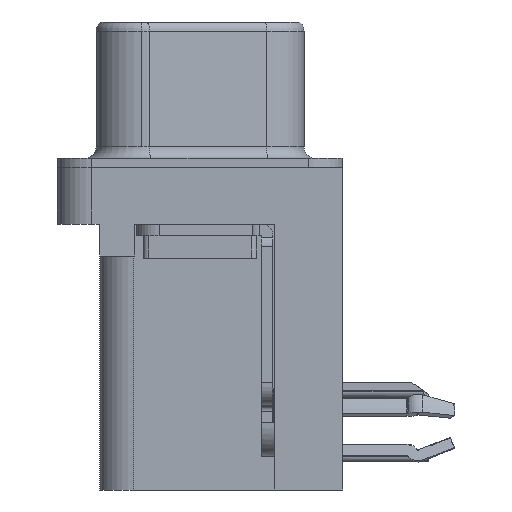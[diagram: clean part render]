
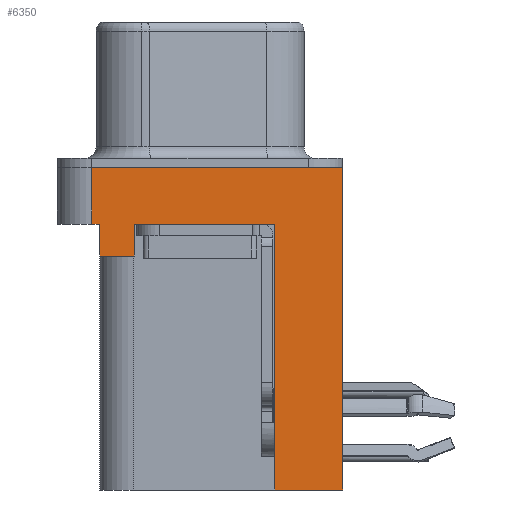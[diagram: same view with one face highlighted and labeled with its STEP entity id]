
A CAD part, left-side view. The second image highlights one B-rep face of the part: STEP entity #6350.
In plain terms, the highlighted planar face has unit normal (-1, 0, 0).
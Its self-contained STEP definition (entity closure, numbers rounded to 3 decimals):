
#9 = VECTOR ( 'NONE', #6792, 1000. ) ;
#83 = VECTOR ( 'NONE', #28165, 1000. ) ;
#802 = ORIENTED_EDGE ( 'NONE', *, *, #1730, .F. ) ;
#912 = DIRECTION ( 'NONE',  ( 0., 0., 1. ) ) ;
#996 = VECTOR ( 'NONE', #2205, 1000. ) ;
#1730 = EDGE_CURVE ( 'NONE', #5535, #6519, #18132, .T. ) ;
#1905 = VERTEX_POINT ( 'NONE', #10035 ) ;
#2050 = VECTOR ( 'NONE', #21379, 1000. ) ;
#2205 = DIRECTION ( 'NONE',  ( 0., 0., 1. ) ) ;
#2220 = ORIENTED_EDGE ( 'NONE', *, *, #10463, .F. ) ;
#2523 = CARTESIAN_POINT ( 'NONE',  ( -2.91, -6.275, -2.5 ) ) ;
#2589 = VECTOR ( 'NONE', #27114, 1000. ) ;
#3514 = EDGE_CURVE ( 'NONE', #9556, #25542, #28544, .T. ) ;
#4251 = CARTESIAN_POINT ( 'NONE',  ( -2.91, 2.895, -3.9 ) ) ;
#4475 = EDGE_CURVE ( 'NONE', #10401, #25542, #5679, .T. ) ;
#4551 = DIRECTION ( 'NONE',  ( -1., 0., 0. ) ) ;
#4852 = VECTOR ( 'NONE', #25044, 1000. ) ;
#5535 = VERTEX_POINT ( 'NONE', #4251 ) ;
#5679 = LINE ( 'NONE', #17106, #11137 ) ;
#5737 = VECTOR ( 'NONE', #26136, 1000. ) ;
#5828 = EDGE_CURVE ( 'NONE', #21570, #10401, #19045, .T. ) ;
#6350 = ADVANCED_FACE ( 'NONE', ( #22339 ), #6562, .T. ) ;
#6415 = DIRECTION ( 'NONE',  ( 0., 0., 1. ) ) ;
#6519 = VERTEX_POINT ( 'NONE', #11495 ) ;
#6562 = PLANE ( 'NONE',  #12569 ) ;
#6792 = DIRECTION ( 'NONE',  ( 0., 1., 0. ) ) ;
#6856 = CARTESIAN_POINT ( 'NONE',  ( -2.91, -6.275, -2.5 ) ) ;
#8208 = LINE ( 'NONE', #27894, #2050 ) ;
#9449 = ORIENTED_EDGE ( 'NONE', *, *, #3514, .T. ) ;
#9556 = VERTEX_POINT ( 'NONE', #10599 ) ;
#9736 = CARTESIAN_POINT ( 'NONE',  ( -2.91, 2.895, -3.9 ) ) ;
#10035 = CARTESIAN_POINT ( 'NONE',  ( -2.91, -3.295, -14.2 ) ) ;
#10401 = VERTEX_POINT ( 'NONE', #12692 ) ;
#10463 = EDGE_CURVE ( 'NONE', #1905, #11185, #8208, .T. ) ;
#10571 = EDGE_CURVE ( 'NONE', #6519, #11316, #28325, .T. ) ;
#10599 = CARTESIAN_POINT ( 'NONE',  ( -2.91, -6.275, -14.2 ) ) ;
#11058 = LINE ( 'NONE', #6856, #21261 ) ;
#11137 = VECTOR ( 'NONE', #14369, 1000. ) ;
#11185 = VERTEX_POINT ( 'NONE', #17406 ) ;
#11316 = VERTEX_POINT ( 'NONE', #15526 ) ;
#11495 = CARTESIAN_POINT ( 'NONE',  ( -2.91, 4.425, -3.9 ) ) ;
#11785 = ORIENTED_EDGE ( 'NONE', *, *, #21209, .F. ) ;
#12230 = ORIENTED_EDGE ( 'NONE', *, *, #15459, .T. ) ;
#12569 = AXIS2_PLACEMENT_3D ( 'NONE', #2523, #4551, #6415 ) ;
#12682 = EDGE_CURVE ( 'NONE', #5535, #16068, #20725, .T. ) ;
#12692 = CARTESIAN_POINT ( 'NONE',  ( -2.91, 4.775, 0. ) ) ;
#14079 = CARTESIAN_POINT ( 'NONE',  ( -2.91, 4.425, -3.9 ) ) ;
#14369 = DIRECTION ( 'NONE',  ( 0., -1., 0. ) ) ;
#14659 = ORIENTED_EDGE ( 'NONE', *, *, #5828, .F. ) ;
#15435 = CARTESIAN_POINT ( 'NONE',  ( -2.91, 4.775, -2.5 ) ) ;
#15459 = EDGE_CURVE ( 'NONE', #21570, #11316, #26543, .T. ) ;
#15526 = CARTESIAN_POINT ( 'NONE',  ( -2.91, 4.425, -2.5 ) ) ;
#15677 = DIRECTION ( 'NONE',  ( 0., -1., 0. ) ) ;
#16068 = VERTEX_POINT ( 'NONE', #18795 ) ;
#17106 = CARTESIAN_POINT ( 'NONE',  ( -2.91, -6.275, 0. ) ) ;
#17406 = CARTESIAN_POINT ( 'NONE',  ( -2.91, -3.295, -2.5 ) ) ;
#17553 = ORIENTED_EDGE ( 'NONE', *, *, #20933, .T. ) ;
#17776 = CARTESIAN_POINT ( 'NONE',  ( -2.91, -3.295, -14.2 ) ) ;
#17925 = LINE ( 'NONE', #17776, #9 ) ;
#18132 = LINE ( 'NONE', #14079, #2589 ) ;
#18795 = CARTESIAN_POINT ( 'NONE',  ( -2.91, 2.895, -2.5 ) ) ;
#19045 = LINE ( 'NONE', #25690, #83 ) ;
#20041 = CARTESIAN_POINT ( 'NONE',  ( -2.91, -6.275, -2.5 ) ) ;
#20725 = LINE ( 'NONE', #9736, #28013 ) ;
#20895 = ORIENTED_EDGE ( 'NONE', *, *, #10571, .F. ) ;
#20933 = EDGE_CURVE ( 'NONE', #16068, #11185, #11058, .T. ) ;
#21209 = EDGE_CURVE ( 'NONE', #9556, #1905, #17925, .T. ) ;
#21261 = VECTOR ( 'NONE', #15677, 1000. ) ;
#21329 = ORIENTED_EDGE ( 'NONE', *, *, #4475, .F. ) ;
#21379 = DIRECTION ( 'NONE',  ( 0., 0., 1. ) ) ;
#21523 = EDGE_LOOP ( 'NONE', ( #21329, #14659, #12230, #20895, #802, #26496, #17553, #2220, #11785, #9449 ) ) ;
#21570 = VERTEX_POINT ( 'NONE', #15435 ) ;
#22025 = CARTESIAN_POINT ( 'NONE',  ( -2.91, -6.275, -2.5 ) ) ;
#22339 = FACE_OUTER_BOUND ( 'NONE', #21523, .T. ) ;
#25044 = DIRECTION ( 'NONE',  ( 0., -1., 0. ) ) ;
#25542 = VERTEX_POINT ( 'NONE', #25866 ) ;
#25690 = CARTESIAN_POINT ( 'NONE',  ( -2.91, 4.775, -2.5 ) ) ;
#25866 = CARTESIAN_POINT ( 'NONE',  ( -2.91, -6.275, 0. ) ) ;
#26136 = DIRECTION ( 'NONE',  ( 0., 0., 1. ) ) ;
#26496 = ORIENTED_EDGE ( 'NONE', *, *, #12682, .T. ) ;
#26543 = LINE ( 'NONE', #20041, #4852 ) ;
#26573 = CARTESIAN_POINT ( 'NONE',  ( -2.91, 4.425, -3.9 ) ) ;
#27114 = DIRECTION ( 'NONE',  ( 0., 1., 0. ) ) ;
#27894 = CARTESIAN_POINT ( 'NONE',  ( -2.91, -3.295, -14.2 ) ) ;
#28013 = VECTOR ( 'NONE', #912, 1000. ) ;
#28165 = DIRECTION ( 'NONE',  ( 0., 0., 1. ) ) ;
#28325 = LINE ( 'NONE', #26573, #5737 ) ;
#28544 = LINE ( 'NONE', #22025, #996 ) ;
